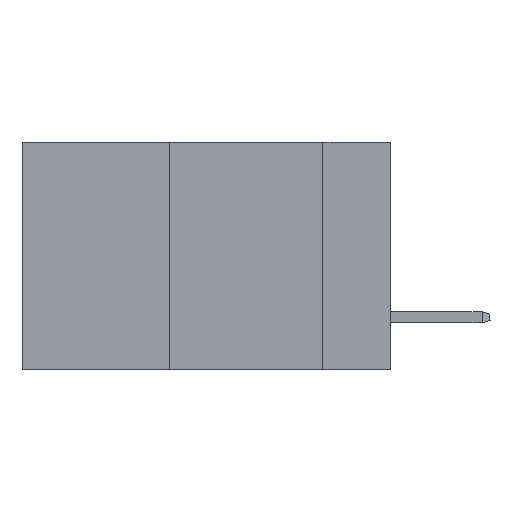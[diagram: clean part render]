
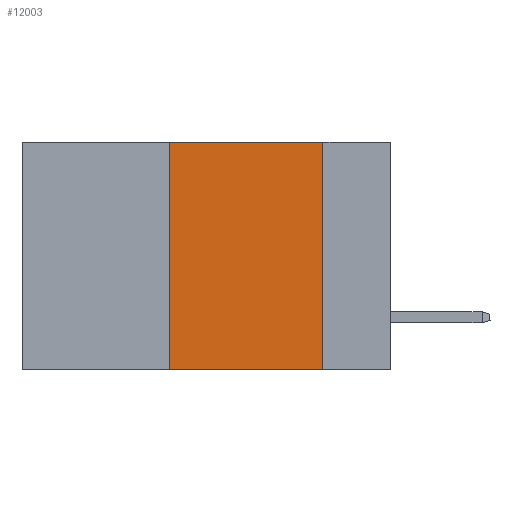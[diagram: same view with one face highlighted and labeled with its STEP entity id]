
A CAD part, left-side view. The second image highlights one B-rep face of the part: STEP entity #12003.
In plain terms, the highlighted planar face has unit normal (-1, 0, 0).
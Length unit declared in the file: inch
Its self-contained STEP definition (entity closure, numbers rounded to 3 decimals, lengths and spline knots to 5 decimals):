
#144 = FACE_OUTER_BOUND ( 'NONE', #12895, .T. ) ;
#284 = ORIENTED_EDGE ( 'NONE', *, *, #15078, .F. ) ;
#584 = VERTEX_POINT ( 'NONE', #20034 ) ;
#1882 = AXIS2_PLACEMENT_3D ( 'NONE', #8470, #22218, #10448 ) ;
#2381 = DIRECTION ( 'NONE',  ( 0., -1., 0. ) ) ;
#2412 = LINE ( 'NONE', #6397, #7182 ) ;
#2986 = VECTOR ( 'NONE', #14511, 39.37008 ) ;
#3133 = CARTESIAN_POINT ( 'NONE',  ( 0., 0.36, 0. ) ) ;
#3225 = CARTESIAN_POINT ( 'NONE',  ( 0., 0.36, -0.37 ) ) ;
#3451 = VECTOR ( 'NONE', #4442, 39.37008 ) ;
#4078 = LINE ( 'NONE', #14289, #3451 ) ;
#4256 = VERTEX_POINT ( 'NONE', #16707 ) ;
#4442 = DIRECTION ( 'NONE',  ( 0., -1., 0. ) ) ;
#4474 = PLANE ( 'NONE',  #1882 ) ;
#4667 = CARTESIAN_POINT ( 'NONE',  ( 0., 0.11, 0. ) ) ;
#5516 = CARTESIAN_POINT ( 'NONE',  ( 0., 0.36, 0. ) ) ;
#6397 = CARTESIAN_POINT ( 'NONE',  ( 0., 0.6, -0.37 ) ) ;
#6668 = EDGE_CURVE ( 'NONE', #22943, #19348, #19594, .T. ) ;
#7182 = VECTOR ( 'NONE', #2381, 39.37008 ) ;
#8470 = CARTESIAN_POINT ( 'NONE',  ( 0., 0.6, 0. ) ) ;
#8766 = EDGE_CURVE ( 'NONE', #19348, #4256, #4078, .T. ) ;
#9546 = LINE ( 'NONE', #4667, #2986 ) ;
#10448 = DIRECTION ( 'NONE',  ( 0., 0., -1. ) ) ;
#10951 = ORIENTED_EDGE ( 'NONE', *, *, #8766, .F. ) ;
#12003 = ADVANCED_FACE ( 'NONE', ( #144 ), #4474, .F. ) ;
#12895 = EDGE_LOOP ( 'NONE', ( #284, #10951, #20167, #25380 ) ) ;
#14289 = CARTESIAN_POINT ( 'NONE',  ( 0., 0.6, 0. ) ) ;
#14511 = DIRECTION ( 'NONE',  ( 0., 0., -1. ) ) ;
#15078 = EDGE_CURVE ( 'NONE', #4256, #584, #9546, .T. ) ;
#16707 = CARTESIAN_POINT ( 'NONE',  ( 0., 0.11, 0. ) ) ;
#19348 = VERTEX_POINT ( 'NONE', #5516 ) ;
#19594 = LINE ( 'NONE', #3133, #24793 ) ;
#20034 = CARTESIAN_POINT ( 'NONE',  ( 0., 0.11, -0.37 ) ) ;
#20167 = ORIENTED_EDGE ( 'NONE', *, *, #6668, .F. ) ;
#22218 = DIRECTION ( 'NONE',  ( 1., 0., 0. ) ) ;
#22943 = VERTEX_POINT ( 'NONE', #3225 ) ;
#24793 = VECTOR ( 'NONE', #25049, 39.37008 ) ;
#25049 = DIRECTION ( 'NONE',  ( 0., 0., 1. ) ) ;
#25068 = EDGE_CURVE ( 'NONE', #22943, #584, #2412, .T. ) ;
#25380 = ORIENTED_EDGE ( 'NONE', *, *, #25068, .T. ) ;
